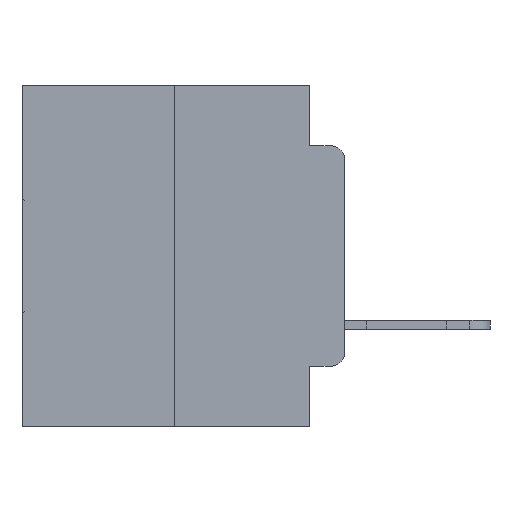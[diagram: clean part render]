
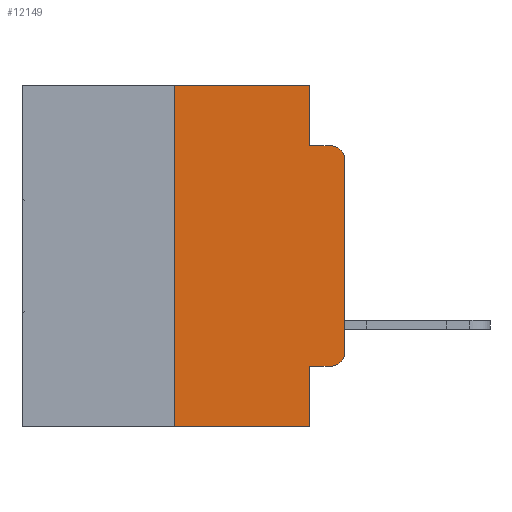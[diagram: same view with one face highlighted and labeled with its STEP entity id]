
A CAD part, left-side view. The second image highlights one B-rep face of the part: STEP entity #12149.
In plain terms, the highlighted planar face has unit normal (-1, 0, 0).
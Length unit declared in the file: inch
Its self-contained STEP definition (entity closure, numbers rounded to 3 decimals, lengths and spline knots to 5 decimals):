
#187 = CARTESIAN_POINT ( 'NONE',  ( 0., 0.051, 0. ) ) ;
#226 = VERTEX_POINT ( 'NONE', #4107 ) ;
#264 = DIRECTION ( 'NONE',  ( -1., 0., 0. ) ) ;
#321 = EDGE_LOOP ( 'NONE', ( #9282, #29211, #16822, #16871, #2107, #10727, #1408, #1723, #1917, #2266 ) ) ;
#638 = CARTESIAN_POINT ( 'NONE',  ( 0., 0.25, 0. ) ) ;
#868 = CARTESIAN_POINT ( 'NONE',  ( 0., 0.25, -0.5 ) ) ;
#1397 = DIRECTION ( 'NONE',  ( 0., 0., 1. ) ) ;
#1408 = ORIENTED_EDGE ( 'NONE', *, *, #11706, .T. ) ;
#1723 = ORIENTED_EDGE ( 'NONE', *, *, #16745, .F. ) ;
#1917 = ORIENTED_EDGE ( 'NONE', *, *, #12477, .T. ) ;
#2107 = ORIENTED_EDGE ( 'NONE', *, *, #23841, .F. ) ;
#2266 = ORIENTED_EDGE ( 'NONE', *, *, #12879, .T. ) ;
#2720 = DIRECTION ( 'NONE',  ( 0., 0., -1. ) ) ;
#2909 = DIRECTION ( 'NONE',  ( 0., -1., 0. ) ) ;
#3170 = DIRECTION ( 'NONE',  ( 0., 0., 1. ) ) ;
#3545 = LINE ( 'NONE', #11319, #20735 ) ;
#3652 = DIRECTION ( 'NONE',  ( 0., -1., 0. ) ) ;
#3814 = VERTEX_POINT ( 'NONE', #9469 ) ;
#4084 = CARTESIAN_POINT ( 'NONE',  ( 0., 0.02, -0.0885 ) ) ;
#4107 = CARTESIAN_POINT ( 'NONE',  ( 0., 0.051, 0. ) ) ;
#4471 = VERTEX_POINT ( 'NONE', #20926 ) ;
#4588 = CARTESIAN_POINT ( 'NONE',  ( 0., 0.473, 0. ) ) ;
#4631 = CIRCLE ( 'NONE', #13405, 0.02 ) ;
#4993 = LINE ( 'NONE', #22174, #28389 ) ;
#6005 = VERTEX_POINT ( 'NONE', #26563 ) ;
#6219 = CARTESIAN_POINT ( 'NONE',  ( 0., 0., -0.1085 ) ) ;
#6925 = DIRECTION ( 'NONE',  ( 0., 0., -1. ) ) ;
#8220 = VECTOR ( 'NONE', #2909, 39.37008 ) ;
#8398 = VERTEX_POINT ( 'NONE', #14019 ) ;
#9282 = ORIENTED_EDGE ( 'NONE', *, *, #20921, .T. ) ;
#9469 = CARTESIAN_POINT ( 'NONE',  ( 0., 0.25, 0. ) ) ;
#9509 = FACE_OUTER_BOUND ( 'NONE', #321, .T. ) ;
#9598 = VERTEX_POINT ( 'NONE', #868 ) ;
#10203 = LINE ( 'NONE', #13141, #21735 ) ;
#10727 = ORIENTED_EDGE ( 'NONE', *, *, #22547, .F. ) ;
#10776 = DIRECTION ( 'NONE',  ( 0., -1., 0. ) ) ;
#11310 = EDGE_CURVE ( 'NONE', #19255, #27773, #24176, .T. ) ;
#11319 = CARTESIAN_POINT ( 'NONE',  ( 0., 0.051, 0. ) ) ;
#11706 = EDGE_CURVE ( 'NONE', #9598, #17105, #25521, .T. ) ;
#12149 = ADVANCED_FACE ( 'NONE', ( #9509 ), #29388, .F. ) ;
#12477 = EDGE_CURVE ( 'NONE', #13713, #8398, #10203, .T. ) ;
#12879 = EDGE_CURVE ( 'NONE', #8398, #6005, #4631, .T. ) ;
#13069 = EDGE_CURVE ( 'NONE', #4471, #27773, #4993, .T. ) ;
#13141 = CARTESIAN_POINT ( 'NONE',  ( 0., 0.051, -0.4115 ) ) ;
#13314 = DIRECTION ( 'NONE',  ( -1., 0., 0. ) ) ;
#13405 = AXIS2_PLACEMENT_3D ( 'NONE', #14651, #264, #16948 ) ;
#13683 = DIRECTION ( 'NONE',  ( 0., 0., -1. ) ) ;
#13713 = VERTEX_POINT ( 'NONE', #28945 ) ;
#14019 = CARTESIAN_POINT ( 'NONE',  ( 0., 0.02, -0.4115 ) ) ;
#14623 = CARTESIAN_POINT ( 'NONE',  ( 0., 0.473, -0.5 ) ) ;
#14651 = CARTESIAN_POINT ( 'NONE',  ( 0., 0.02, -0.3915 ) ) ;
#14852 = CARTESIAN_POINT ( 'NONE',  ( 0., 0.473, 0. ) ) ;
#15567 = CARTESIAN_POINT ( 'NONE',  ( 0., 0., 0. ) ) ;
#16499 = EDGE_CURVE ( 'NONE', #226, #4471, #3545, .T. ) ;
#16600 = LINE ( 'NONE', #15567, #20519 ) ;
#16745 = EDGE_CURVE ( 'NONE', #13713, #17105, #27493, .T. ) ;
#16822 = ORIENTED_EDGE ( 'NONE', *, *, #13069, .F. ) ;
#16871 = ORIENTED_EDGE ( 'NONE', *, *, #16499, .F. ) ;
#16948 = DIRECTION ( 'NONE',  ( 0., 0., -1. ) ) ;
#17031 = DIRECTION ( 'NONE',  ( 0., -1., 0. ) ) ;
#17105 = VERTEX_POINT ( 'NONE', #24736 ) ;
#19255 = VERTEX_POINT ( 'NONE', #6219 ) ;
#19678 = VECTOR ( 'NONE', #17031, 39.37008 ) ;
#20355 = VECTOR ( 'NONE', #2720, 39.37008 ) ;
#20519 = VECTOR ( 'NONE', #1397, 39.37008 ) ;
#20735 = VECTOR ( 'NONE', #13683, 39.37008 ) ;
#20869 = DIRECTION ( 'NONE',  ( 1., 0., 0. ) ) ;
#20921 = EDGE_CURVE ( 'NONE', #6005, #19255, #16600, .T. ) ;
#20926 = CARTESIAN_POINT ( 'NONE',  ( 0., 0.051, -0.0885 ) ) ;
#21735 = VECTOR ( 'NONE', #10776, 39.37008 ) ;
#22174 = CARTESIAN_POINT ( 'NONE',  ( 0., 0.051, -0.0885 ) ) ;
#22547 = EDGE_CURVE ( 'NONE', #9598, #3814, #25465, .T. ) ;
#23423 = VECTOR ( 'NONE', #3170, 39.37008 ) ;
#23841 = EDGE_CURVE ( 'NONE', #3814, #226, #26379, .T. ) ;
#24154 = AXIS2_PLACEMENT_3D ( 'NONE', #4588, #20869, #6925 ) ;
#24176 = CIRCLE ( 'NONE', #24314, 0.02 ) ;
#24314 = AXIS2_PLACEMENT_3D ( 'NONE', #26706, #13314, #28799 ) ;
#24736 = CARTESIAN_POINT ( 'NONE',  ( 0., 0.051, -0.5 ) ) ;
#25465 = LINE ( 'NONE', #638, #23423 ) ;
#25521 = LINE ( 'NONE', #14623, #19678 ) ;
#26379 = LINE ( 'NONE', #14852, #8220 ) ;
#26563 = CARTESIAN_POINT ( 'NONE',  ( 0., 0., -0.3915 ) ) ;
#26706 = CARTESIAN_POINT ( 'NONE',  ( 0., 0.02, -0.1085 ) ) ;
#27493 = LINE ( 'NONE', #187, #20355 ) ;
#27773 = VERTEX_POINT ( 'NONE', #4084 ) ;
#28389 = VECTOR ( 'NONE', #3652, 39.37008 ) ;
#28799 = DIRECTION ( 'NONE',  ( 0., 0., -1. ) ) ;
#28945 = CARTESIAN_POINT ( 'NONE',  ( 0., 0.051, -0.4115 ) ) ;
#29211 = ORIENTED_EDGE ( 'NONE', *, *, #11310, .T. ) ;
#29388 = PLANE ( 'NONE',  #24154 ) ;
